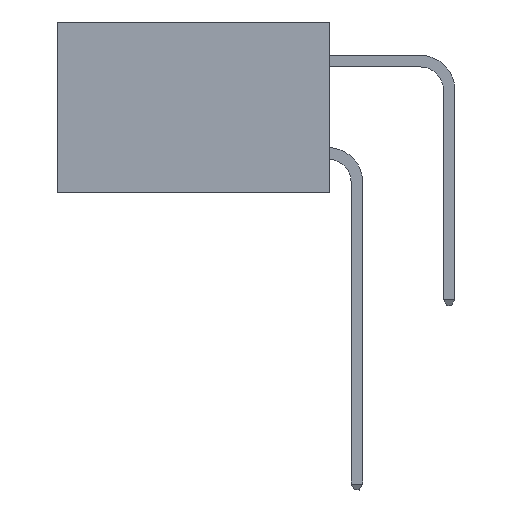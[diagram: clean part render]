
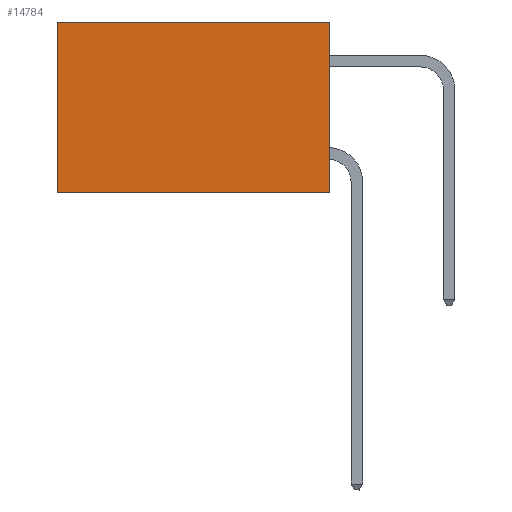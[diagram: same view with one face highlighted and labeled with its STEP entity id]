
A CAD part, left-side view. The second image highlights one B-rep face of the part: STEP entity #14784.
In plain terms, the highlighted planar face has unit normal (-1, 0, 0).
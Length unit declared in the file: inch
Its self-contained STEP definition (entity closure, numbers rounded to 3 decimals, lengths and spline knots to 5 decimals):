
#810 = AXIS2_PLACEMENT_3D ( 'NONE', #20879, #30908, #15898 ) ;
#1713 = DIRECTION ( 'NONE',  ( 0., 1., 0. ) ) ;
#2536 = VERTEX_POINT ( 'NONE', #14044 ) ;
#4280 = ORIENTED_EDGE ( 'NONE', *, *, #18994, .F. ) ;
#5047 = LINE ( 'NONE', #31076, #10949 ) ;
#6551 = VERTEX_POINT ( 'NONE', #25003 ) ;
#7549 = EDGE_CURVE ( 'NONE', #26876, #12009, #26520, .T. ) ;
#8581 = LINE ( 'NONE', #29311, #27803 ) ;
#8708 = ORIENTED_EDGE ( 'NONE', *, *, #13462, .T. ) ;
#9954 = DIRECTION ( 'NONE',  ( 0., 0., -1. ) ) ;
#10300 = VECTOR ( 'NONE', #9954, 39.37008 ) ;
#10949 = VECTOR ( 'NONE', #18583, 39.37008 ) ;
#11396 = EDGE_LOOP ( 'NONE', ( #12214, #25937, #4280, #8708 ) ) ;
#11923 = DIRECTION ( 'NONE',  ( 0., 1., 0. ) ) ;
#11960 = CARTESIAN_POINT ( 'NONE',  ( 0.277, 0., -0.37 ) ) ;
#12009 = VERTEX_POINT ( 'NONE', #31003 ) ;
#12214 = ORIENTED_EDGE ( 'NONE', *, *, #17207, .T. ) ;
#13462 = EDGE_CURVE ( 'NONE', #6551, #2536, #8581, .T. ) ;
#14044 = CARTESIAN_POINT ( 'NONE',  ( 0.277, 0.59, 0. ) ) ;
#14784 = ADVANCED_FACE ( 'NONE', ( #29287 ), #28398, .F. ) ;
#15898 = DIRECTION ( 'NONE',  ( 0., 0., -1. ) ) ;
#17207 = EDGE_CURVE ( 'NONE', #2536, #12009, #29524, .T. ) ;
#17512 = CARTESIAN_POINT ( 'NONE',  ( 0.277, 0.59, -0.37 ) ) ;
#18583 = DIRECTION ( 'NONE',  ( 0., 0., -1. ) ) ;
#18994 = EDGE_CURVE ( 'NONE', #6551, #26876, #5047, .T. ) ;
#20879 = CARTESIAN_POINT ( 'NONE',  ( 0.277, 0., -0.37 ) ) ;
#21006 = CARTESIAN_POINT ( 'NONE',  ( 0.277, 0., -0.37 ) ) ;
#25003 = CARTESIAN_POINT ( 'NONE',  ( 0.277, 0., 0. ) ) ;
#25937 = ORIENTED_EDGE ( 'NONE', *, *, #7549, .F. ) ;
#26520 = LINE ( 'NONE', #11960, #27300 ) ;
#26876 = VERTEX_POINT ( 'NONE', #21006 ) ;
#27300 = VECTOR ( 'NONE', #11923, 39.37008 ) ;
#27803 = VECTOR ( 'NONE', #1713, 39.37008 ) ;
#28398 = PLANE ( 'NONE',  #810 ) ;
#29287 = FACE_OUTER_BOUND ( 'NONE', #11396, .T. ) ;
#29311 = CARTESIAN_POINT ( 'NONE',  ( 0.277, 0., 0. ) ) ;
#29524 = LINE ( 'NONE', #17512, #10300 ) ;
#30908 = DIRECTION ( 'NONE',  ( 1., 0., 0. ) ) ;
#31003 = CARTESIAN_POINT ( 'NONE',  ( 0.277, 0.59, -0.37 ) ) ;
#31076 = CARTESIAN_POINT ( 'NONE',  ( 0.277, 0., -0.37 ) ) ;
